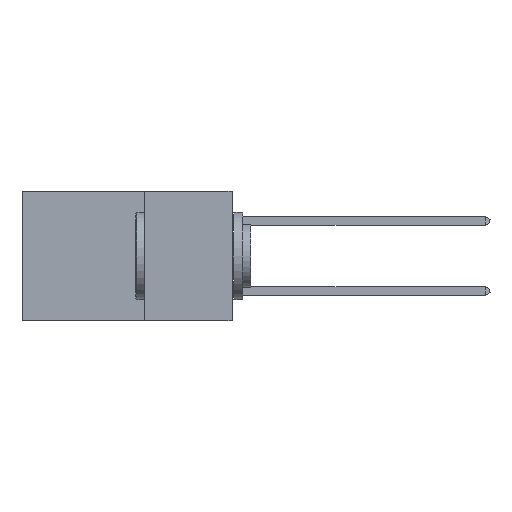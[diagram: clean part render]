
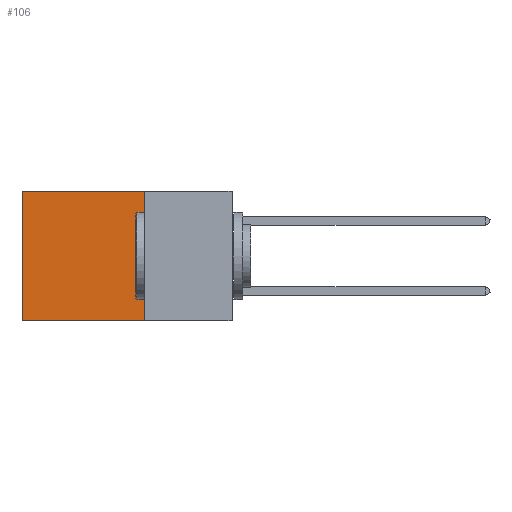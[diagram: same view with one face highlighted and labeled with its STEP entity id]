
A CAD part, left-side view. The second image highlights one B-rep face of the part: STEP entity #106.
In plain terms, the highlighted planar face has unit normal (-1, 0, 0).
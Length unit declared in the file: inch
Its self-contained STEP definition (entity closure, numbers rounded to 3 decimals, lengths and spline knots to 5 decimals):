
#106 = ADVANCED_FACE ( 'NONE', ( #13318 ), #33798, .F. ) ;
#360 = LINE ( 'NONE', #7765, #28663 ) ;
#5072 = DIRECTION ( 'NONE',  ( 1., 0., 0. ) ) ;
#5593 = EDGE_CURVE ( 'NONE', #44580, #25043, #360, .T. ) ;
#6628 = VERTEX_POINT ( 'NONE', #14266 ) ;
#7765 = CARTESIAN_POINT ( 'NONE',  ( 0.2875, 0.25, 0. ) ) ;
#13318 = FACE_OUTER_BOUND ( 'NONE', #31358, .T. ) ;
#13666 = VECTOR ( 'NONE', #37268, 39.37008 ) ;
#14142 = ORIENTED_EDGE ( 'NONE', *, *, #30058, .T. ) ;
#14266 = CARTESIAN_POINT ( 'NONE',  ( 0.2875, 0.6, -0.37 ) ) ;
#15824 = EDGE_CURVE ( 'NONE', #44580, #38352, #37271, .T. ) ;
#16661 = CARTESIAN_POINT ( 'NONE',  ( 0.2875, 0.6, 0. ) ) ;
#16880 = VECTOR ( 'NONE', #46590, 39.37008 ) ;
#21953 = LINE ( 'NONE', #45961, #29970 ) ;
#23259 = ORIENTED_EDGE ( 'NONE', *, *, #5593, .T. ) ;
#25043 = VERTEX_POINT ( 'NONE', #16661 ) ;
#25867 = DIRECTION ( 'NONE',  ( 0., 1., 0. ) ) ;
#26546 = AXIS2_PLACEMENT_3D ( 'NONE', #34922, #5072, #30882 ) ;
#27288 = CARTESIAN_POINT ( 'NONE',  ( 0.2875, 0.25, 0. ) ) ;
#27832 = LINE ( 'NONE', #31807, #16880 ) ;
#28663 = VECTOR ( 'NONE', #25867, 39.37008 ) ;
#29970 = VECTOR ( 'NONE', #46111, 39.37008 ) ;
#30058 = EDGE_CURVE ( 'NONE', #25043, #6628, #27832, .T. ) ;
#30882 = DIRECTION ( 'NONE',  ( 0., 0., -1. ) ) ;
#31358 = EDGE_LOOP ( 'NONE', ( #14142, #38823, #45113, #23259 ) ) ;
#31807 = CARTESIAN_POINT ( 'NONE',  ( 0.2875, 0.6, 0. ) ) ;
#31945 = EDGE_CURVE ( 'NONE', #38352, #6628, #21953, .T. ) ;
#33591 = CARTESIAN_POINT ( 'NONE',  ( 0.2875, 0.25, 0. ) ) ;
#33798 = PLANE ( 'NONE',  #26546 ) ;
#34922 = CARTESIAN_POINT ( 'NONE',  ( 0.2875, 0.25, 0. ) ) ;
#37268 = DIRECTION ( 'NONE',  ( 0., 0., -1. ) ) ;
#37271 = LINE ( 'NONE', #33591, #13666 ) ;
#38352 = VERTEX_POINT ( 'NONE', #44576 ) ;
#38823 = ORIENTED_EDGE ( 'NONE', *, *, #31945, .F. ) ;
#44576 = CARTESIAN_POINT ( 'NONE',  ( 0.2875, 0.25, -0.37 ) ) ;
#44580 = VERTEX_POINT ( 'NONE', #27288 ) ;
#45113 = ORIENTED_EDGE ( 'NONE', *, *, #15824, .F. ) ;
#45961 = CARTESIAN_POINT ( 'NONE',  ( 0.2875, 0.25, -0.37 ) ) ;
#46111 = DIRECTION ( 'NONE',  ( 0., 1., 0. ) ) ;
#46590 = DIRECTION ( 'NONE',  ( 0., 0., -1. ) ) ;
